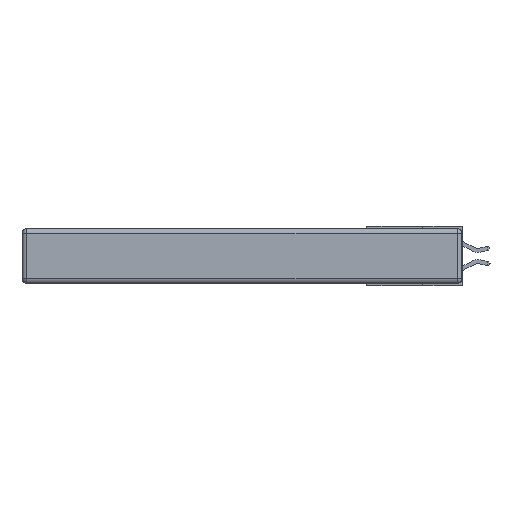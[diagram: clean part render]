
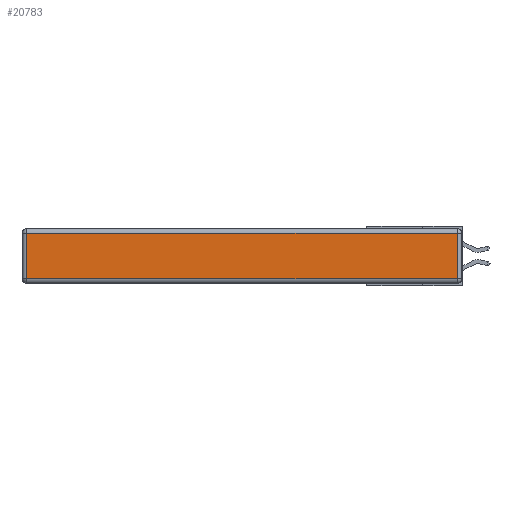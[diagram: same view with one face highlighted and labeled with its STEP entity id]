
A CAD part, left-side view. The second image highlights one B-rep face of the part: STEP entity #20783.
In plain terms, the highlighted planar face has unit normal (-1, 0, 0).
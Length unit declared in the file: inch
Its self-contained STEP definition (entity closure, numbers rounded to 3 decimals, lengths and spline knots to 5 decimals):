
#678 = LINE ( 'NONE', #2876, #5975 ) ;
#1140 = CARTESIAN_POINT ( 'NONE',  ( 0., 2.72, -0.03 ) ) ;
#1876 = DIRECTION ( 'NONE',  ( -1., 0., 0. ) ) ;
#1967 = CARTESIAN_POINT ( 'NONE',  ( 0., 0., -0.313 ) ) ;
#2518 = ORIENTED_EDGE ( 'NONE', *, *, #24731, .T. ) ;
#2876 = CARTESIAN_POINT ( 'NONE',  ( 0., 2.75, -0.03 ) ) ;
#3529 = ORIENTED_EDGE ( 'NONE', *, *, #14539, .T. ) ;
#3637 = DIRECTION ( 'NONE',  ( 0., 0., 1. ) ) ;
#5885 = CARTESIAN_POINT ( 'NONE',  ( 0., 0.03, -0.03 ) ) ;
#5975 = VECTOR ( 'NONE', #8804, 39.37008 ) ;
#7044 = VECTOR ( 'NONE', #3637, 39.37008 ) ;
#7718 = EDGE_LOOP ( 'NONE', ( #2518, #3529, #17067, #8212 ) ) ;
#7799 = VERTEX_POINT ( 'NONE', #13473 ) ;
#8212 = ORIENTED_EDGE ( 'NONE', *, *, #22875, .T. ) ;
#8804 = DIRECTION ( 'NONE',  ( 0., 1., 0. ) ) ;
#9325 = VERTEX_POINT ( 'NONE', #18093 ) ;
#11540 = EDGE_CURVE ( 'NONE', #24710, #19984, #678, .T. ) ;
#12410 = LINE ( 'NONE', #19115, #7044 ) ;
#13473 = CARTESIAN_POINT ( 'NONE',  ( 0., 0.03, -0.313 ) ) ;
#13692 = PLANE ( 'NONE',  #24997 ) ;
#14493 = DIRECTION ( 'NONE',  ( 0., -1., 0. ) ) ;
#14539 = EDGE_CURVE ( 'NONE', #7799, #24710, #12410, .T. ) ;
#17067 = ORIENTED_EDGE ( 'NONE', *, *, #11540, .T. ) ;
#18093 = CARTESIAN_POINT ( 'NONE',  ( 0., 2.72, -0.313 ) ) ;
#18444 = CARTESIAN_POINT ( 'NONE',  ( 0., 2.72, -0.343 ) ) ;
#19115 = CARTESIAN_POINT ( 'NONE',  ( 0., 0.03, -0.343 ) ) ;
#19984 = VERTEX_POINT ( 'NONE', #1140 ) ;
#20416 = DIRECTION ( 'NONE',  ( 0., 0., -1. ) ) ;
#20783 = ADVANCED_FACE ( 'NONE', ( #22704 ), #13692, .T. ) ;
#20924 = VECTOR ( 'NONE', #20416, 39.37008 ) ;
#21223 = LINE ( 'NONE', #18444, #20924 ) ;
#21782 = CARTESIAN_POINT ( 'NONE',  ( 0., 0., -0.343 ) ) ;
#22447 = LINE ( 'NONE', #1967, #24286 ) ;
#22704 = FACE_OUTER_BOUND ( 'NONE', #7718, .T. ) ;
#22875 = EDGE_CURVE ( 'NONE', #19984, #9325, #21223, .T. ) ;
#23710 = DIRECTION ( 'NONE',  ( 0., 0., 1. ) ) ;
#24286 = VECTOR ( 'NONE', #14493, 39.37008 ) ;
#24710 = VERTEX_POINT ( 'NONE', #5885 ) ;
#24731 = EDGE_CURVE ( 'NONE', #9325, #7799, #22447, .T. ) ;
#24997 = AXIS2_PLACEMENT_3D ( 'NONE', #21782, #1876, #23710 ) ;
